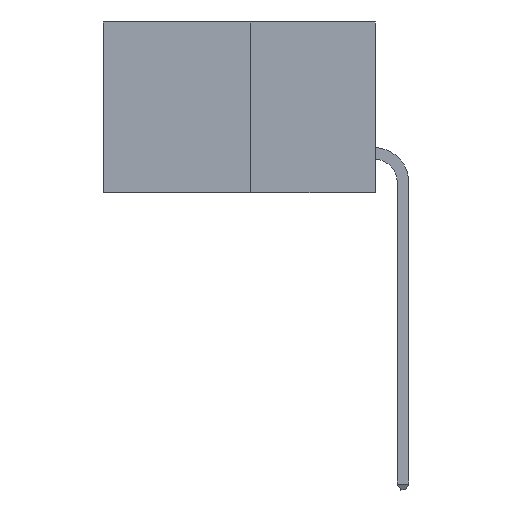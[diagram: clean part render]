
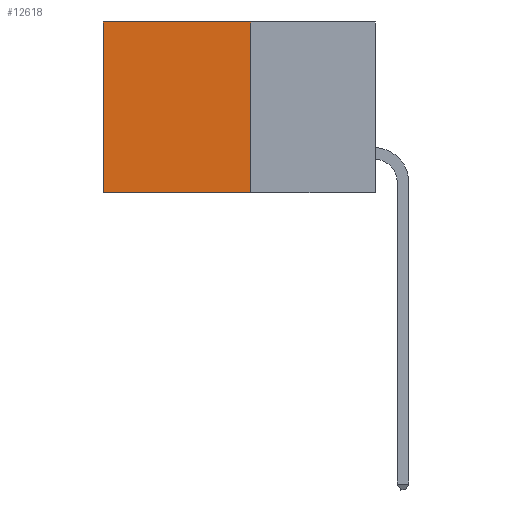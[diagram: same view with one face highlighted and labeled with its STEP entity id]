
A CAD part, left-side view. The second image highlights one B-rep face of the part: STEP entity #12618.
In plain terms, the highlighted planar face has unit normal (-1, 0, 0).
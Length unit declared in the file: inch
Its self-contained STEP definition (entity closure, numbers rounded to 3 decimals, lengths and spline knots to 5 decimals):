
#526 = CARTESIAN_POINT ( 'NONE',  ( 0.277, 0.27, 0. ) ) ;
#895 = DIRECTION ( 'NONE',  ( 0., 1., 0. ) ) ;
#1118 = ORIENTED_EDGE ( 'NONE', *, *, #6649, .T. ) ;
#1383 = VECTOR ( 'NONE', #10114, 39.37008 ) ;
#1959 = VERTEX_POINT ( 'NONE', #12724 ) ;
#2150 = VERTEX_POINT ( 'NONE', #5943 ) ;
#2787 = LINE ( 'NONE', #12538, #13615 ) ;
#3035 = LINE ( 'NONE', #13461, #13864 ) ;
#3706 = PLANE ( 'NONE',  #6150 ) ;
#4515 = LINE ( 'NONE', #5777, #1383 ) ;
#4535 = VERTEX_POINT ( 'NONE', #4835 ) ;
#4744 = DIRECTION ( 'NONE',  ( 1., 0., 0. ) ) ;
#4835 = CARTESIAN_POINT ( 'NONE',  ( 0.277, 0.59, -0.37 ) ) ;
#5667 = EDGE_CURVE ( 'NONE', #7950, #2150, #3035, .T. ) ;
#5777 = CARTESIAN_POINT ( 'NONE',  ( 0.277, 0.27, 0. ) ) ;
#5943 = CARTESIAN_POINT ( 'NONE',  ( 0.277, 0.27, -0.37 ) ) ;
#6150 = AXIS2_PLACEMENT_3D ( 'NONE', #11181, #4744, #12199 ) ;
#6208 = DIRECTION ( 'NONE',  ( 0., 0., -1. ) ) ;
#6649 = EDGE_CURVE ( 'NONE', #1959, #4535, #2787, .T. ) ;
#7379 = CARTESIAN_POINT ( 'NONE',  ( 0.277, 0.27, -0.37 ) ) ;
#7675 = ORIENTED_EDGE ( 'NONE', *, *, #8520, .T. ) ;
#7950 = VERTEX_POINT ( 'NONE', #526 ) ;
#7967 = FACE_OUTER_BOUND ( 'NONE', #12032, .T. ) ;
#8412 = ORIENTED_EDGE ( 'NONE', *, *, #13935, .F. ) ;
#8520 = EDGE_CURVE ( 'NONE', #7950, #1959, #4515, .T. ) ;
#8730 = ORIENTED_EDGE ( 'NONE', *, *, #5667, .F. ) ;
#10114 = DIRECTION ( 'NONE',  ( 0., 1., 0. ) ) ;
#10453 = LINE ( 'NONE', #7379, #12803 ) ;
#11181 = CARTESIAN_POINT ( 'NONE',  ( 0.277, 0.27, -0.37 ) ) ;
#12032 = EDGE_LOOP ( 'NONE', ( #1118, #8412, #8730, #7675 ) ) ;
#12199 = DIRECTION ( 'NONE',  ( 0., 0., -1. ) ) ;
#12538 = CARTESIAN_POINT ( 'NONE',  ( 0.277, 0.59, -0.37 ) ) ;
#12618 = ADVANCED_FACE ( 'NONE', ( #7967 ), #3706, .F. ) ;
#12724 = CARTESIAN_POINT ( 'NONE',  ( 0.277, 0.59, 0. ) ) ;
#12803 = VECTOR ( 'NONE', #895, 39.37008 ) ;
#13247 = DIRECTION ( 'NONE',  ( 0., 0., -1. ) ) ;
#13461 = CARTESIAN_POINT ( 'NONE',  ( 0.277, 0.27, -0.37 ) ) ;
#13615 = VECTOR ( 'NONE', #6208, 39.37008 ) ;
#13864 = VECTOR ( 'NONE', #13247, 39.37008 ) ;
#13935 = EDGE_CURVE ( 'NONE', #2150, #4535, #10453, .T. ) ;
